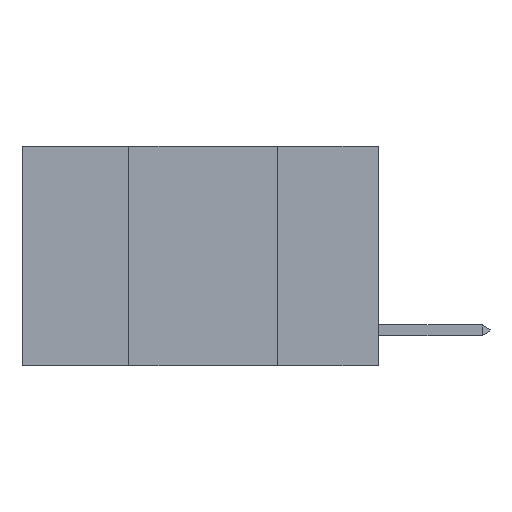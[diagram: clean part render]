
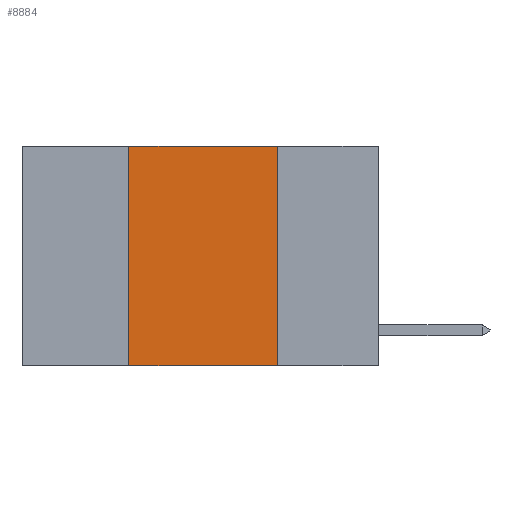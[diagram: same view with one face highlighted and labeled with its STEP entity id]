
A CAD part, left-side view. The second image highlights one B-rep face of the part: STEP entity #8884.
In plain terms, the highlighted planar face has unit normal (-1, 0, 0).
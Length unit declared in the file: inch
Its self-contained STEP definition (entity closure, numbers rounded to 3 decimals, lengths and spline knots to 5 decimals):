
#55 = DIRECTION ( 'NONE',  ( 0., 0., -1. ) ) ;
#272 = ORIENTED_EDGE ( 'NONE', *, *, #11860, .T. ) ;
#887 = LINE ( 'NONE', #2807, #16192 ) ;
#1939 = DIRECTION ( 'NONE',  ( 0., 0., 1. ) ) ;
#2089 = VERTEX_POINT ( 'NONE', #4112 ) ;
#2807 = CARTESIAN_POINT ( 'NONE',  ( 0., 0.6, -0.37 ) ) ;
#2906 = AXIS2_PLACEMENT_3D ( 'NONE', #5750, #16135, #7331 ) ;
#3232 = LINE ( 'NONE', #4511, #3716 ) ;
#3716 = VECTOR ( 'NONE', #55, 39.37008 ) ;
#4112 = CARTESIAN_POINT ( 'NONE',  ( 0., 0.42, 0. ) ) ;
#4511 = CARTESIAN_POINT ( 'NONE',  ( 0., 0.17, 0. ) ) ;
#4826 = VERTEX_POINT ( 'NONE', #5327 ) ;
#4902 = CARTESIAN_POINT ( 'NONE',  ( 0., 0.6, 0. ) ) ;
#4993 = FACE_OUTER_BOUND ( 'NONE', #8531, .T. ) ;
#5327 = CARTESIAN_POINT ( 'NONE',  ( 0., 0.42, -0.37 ) ) ;
#5472 = VERTEX_POINT ( 'NONE', #18697 ) ;
#5750 = CARTESIAN_POINT ( 'NONE',  ( 0., 0.6, 0. ) ) ;
#6629 = EDGE_CURVE ( 'NONE', #2089, #5472, #11419, .T. ) ;
#7331 = DIRECTION ( 'NONE',  ( 0., 0., -1. ) ) ;
#8028 = CARTESIAN_POINT ( 'NONE',  ( 0., 0.17, -0.37 ) ) ;
#8531 = EDGE_LOOP ( 'NONE', ( #14560, #14592, #16924, #272 ) ) ;
#8884 = ADVANCED_FACE ( 'NONE', ( #4993 ), #11693, .F. ) ;
#10863 = CARTESIAN_POINT ( 'NONE',  ( 0., 0.42, 0. ) ) ;
#11325 = EDGE_CURVE ( 'NONE', #5472, #17314, #3232, .T. ) ;
#11419 = LINE ( 'NONE', #4902, #15011 ) ;
#11693 = PLANE ( 'NONE',  #2906 ) ;
#11860 = EDGE_CURVE ( 'NONE', #4826, #17314, #887, .T. ) ;
#12026 = VECTOR ( 'NONE', #1939, 39.37008 ) ;
#12106 = EDGE_CURVE ( 'NONE', #4826, #2089, #15502, .T. ) ;
#13166 = DIRECTION ( 'NONE',  ( 0., -1., 0. ) ) ;
#14560 = ORIENTED_EDGE ( 'NONE', *, *, #11325, .F. ) ;
#14592 = ORIENTED_EDGE ( 'NONE', *, *, #6629, .F. ) ;
#15011 = VECTOR ( 'NONE', #18170, 39.37008 ) ;
#15502 = LINE ( 'NONE', #10863, #12026 ) ;
#16135 = DIRECTION ( 'NONE',  ( 1., 0., 0. ) ) ;
#16192 = VECTOR ( 'NONE', #13166, 39.37008 ) ;
#16924 = ORIENTED_EDGE ( 'NONE', *, *, #12106, .F. ) ;
#17314 = VERTEX_POINT ( 'NONE', #8028 ) ;
#18170 = DIRECTION ( 'NONE',  ( 0., -1., 0. ) ) ;
#18697 = CARTESIAN_POINT ( 'NONE',  ( 0., 0.17, 0. ) ) ;
